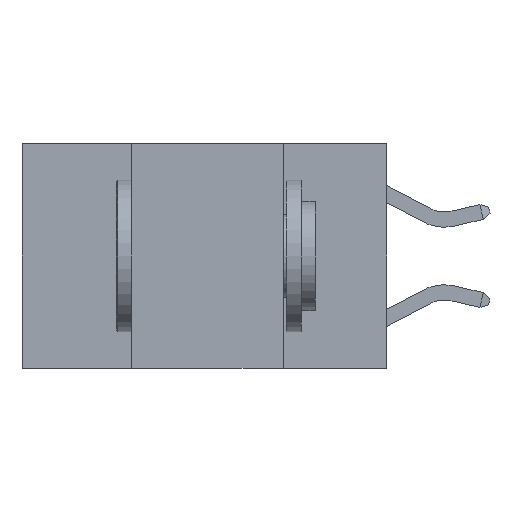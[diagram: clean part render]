
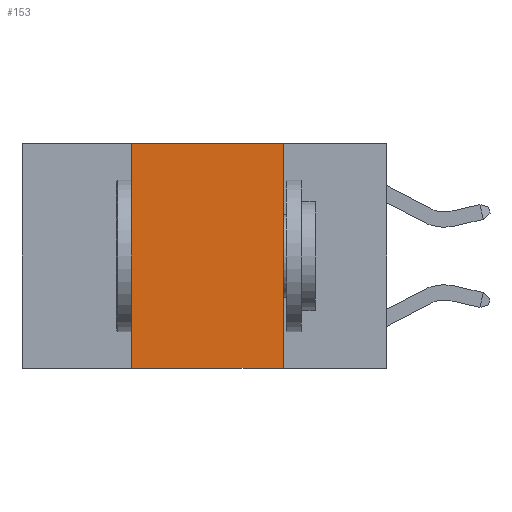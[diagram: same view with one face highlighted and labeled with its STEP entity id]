
A CAD part, left-side view. The second image highlights one B-rep face of the part: STEP entity #153.
In plain terms, the highlighted planar face has unit normal (-1, 0, 0).
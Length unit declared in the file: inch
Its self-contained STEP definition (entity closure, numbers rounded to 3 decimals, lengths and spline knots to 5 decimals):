
#2 = ORIENTED_EDGE ( 'NONE', *, *, #953, .F. ) ;
#153 = ADVANCED_FACE ( 'NONE', ( #913 ), #1572, .F. ) ;
#364 = LINE ( 'NONE', #4105, #5849 ) ;
#885 = LINE ( 'NONE', #8313, #7366 ) ;
#913 = FACE_OUTER_BOUND ( 'NONE', #933, .T. ) ;
#933 = EDGE_LOOP ( 'NONE', ( #8444, #1354, #2, #1534 ) ) ;
#953 = EDGE_CURVE ( 'NONE', #6940, #3963, #364, .T. ) ;
#1354 = ORIENTED_EDGE ( 'NONE', *, *, #3988, .F. ) ;
#1534 = ORIENTED_EDGE ( 'NONE', *, *, #9599, .T. ) ;
#1572 = PLANE ( 'NONE',  #7950 ) ;
#1738 = DIRECTION ( 'NONE',  ( 0., 0., -1. ) ) ;
#2107 = VERTEX_POINT ( 'NONE', #5074 ) ;
#3050 = CARTESIAN_POINT ( 'NONE',  ( 0., 0.6, 0. ) ) ;
#3295 = EDGE_CURVE ( 'NONE', #2107, #9765, #6700, .T. ) ;
#3963 = VERTEX_POINT ( 'NONE', #8007 ) ;
#3988 = EDGE_CURVE ( 'NONE', #3963, #2107, #6036, .T. ) ;
#4105 = CARTESIAN_POINT ( 'NONE',  ( 0., 0.42, 0. ) ) ;
#4699 = DIRECTION ( 'NONE',  ( 0., 0., -1. ) ) ;
#5074 = CARTESIAN_POINT ( 'NONE',  ( 0., 0.17, 0. ) ) ;
#5166 = DIRECTION ( 'NONE',  ( 1., 0., 0. ) ) ;
#5498 = CARTESIAN_POINT ( 'NONE',  ( 0., 0.42, -0.37 ) ) ;
#5849 = VECTOR ( 'NONE', #8454, 39.37008 ) ;
#6036 = LINE ( 'NONE', #3050, #10125 ) ;
#6084 = CARTESIAN_POINT ( 'NONE',  ( 0., 0.17, -0.37 ) ) ;
#6365 = DIRECTION ( 'NONE',  ( 0., -1., 0. ) ) ;
#6700 = LINE ( 'NONE', #10389, #10756 ) ;
#6940 = VERTEX_POINT ( 'NONE', #5498 ) ;
#7366 = VECTOR ( 'NONE', #9127, 39.37008 ) ;
#7950 = AXIS2_PLACEMENT_3D ( 'NONE', #9855, #5166, #1738 ) ;
#8007 = CARTESIAN_POINT ( 'NONE',  ( 0., 0.42, 0. ) ) ;
#8313 = CARTESIAN_POINT ( 'NONE',  ( 0., 0.6, -0.37 ) ) ;
#8444 = ORIENTED_EDGE ( 'NONE', *, *, #3295, .F. ) ;
#8454 = DIRECTION ( 'NONE',  ( 0., 0., 1. ) ) ;
#9127 = DIRECTION ( 'NONE',  ( 0., -1., 0. ) ) ;
#9599 = EDGE_CURVE ( 'NONE', #6940, #9765, #885, .T. ) ;
#9765 = VERTEX_POINT ( 'NONE', #6084 ) ;
#9855 = CARTESIAN_POINT ( 'NONE',  ( 0., 0.6, 0. ) ) ;
#10125 = VECTOR ( 'NONE', #6365, 39.37008 ) ;
#10389 = CARTESIAN_POINT ( 'NONE',  ( 0., 0.17, 0. ) ) ;
#10756 = VECTOR ( 'NONE', #4699, 39.37008 ) ;
